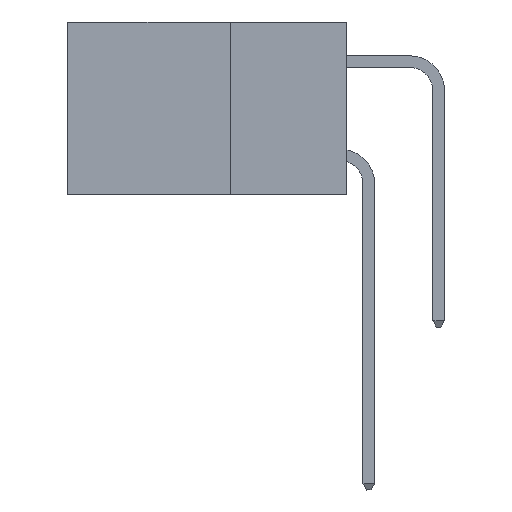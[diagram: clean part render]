
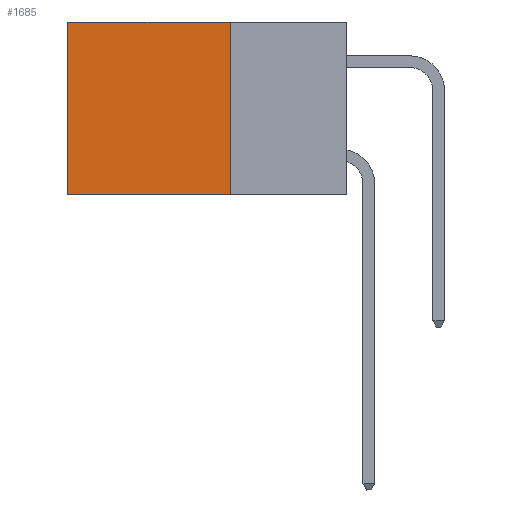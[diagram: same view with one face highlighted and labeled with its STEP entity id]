
A CAD part, left-side view. The second image highlights one B-rep face of the part: STEP entity #1685.
In plain terms, the highlighted planar face has unit normal (-1, 0, 0).
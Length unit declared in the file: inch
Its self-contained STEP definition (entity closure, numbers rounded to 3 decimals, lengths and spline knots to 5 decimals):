
#137 = VERTEX_POINT ( 'NONE', #4758 ) ;
#221 = ORIENTED_EDGE ( 'NONE', *, *, #7578, .F. ) ;
#1452 = CARTESIAN_POINT ( 'NONE',  ( 0.2875, 0.25, -0.37 ) ) ;
#1685 = ADVANCED_FACE ( 'NONE', ( #2567 ), #14187, .F. ) ;
#2338 = CARTESIAN_POINT ( 'NONE',  ( 0.2875, 0.25, 0. ) ) ;
#2486 = DIRECTION ( 'NONE',  ( 0., 0., -1. ) ) ;
#2567 = FACE_OUTER_BOUND ( 'NONE', #16604, .T. ) ;
#3935 = DIRECTION ( 'NONE',  ( 0., 1., 0. ) ) ;
#4029 = CARTESIAN_POINT ( 'NONE',  ( 0.2875, 0.25, 0. ) ) ;
#4758 = CARTESIAN_POINT ( 'NONE',  ( 0.2875, 0.6, 0. ) ) ;
#5301 = LINE ( 'NONE', #1452, #12994 ) ;
#5753 = VECTOR ( 'NONE', #16807, 39.37008 ) ;
#5781 = EDGE_CURVE ( 'NONE', #137, #7153, #13782, .T. ) ;
#5919 = CARTESIAN_POINT ( 'NONE',  ( 0.2875, 0.25, -0.37 ) ) ;
#6412 = EDGE_CURVE ( 'NONE', #6951, #137, #6416, .T. ) ;
#6416 = LINE ( 'NONE', #11622, #5753 ) ;
#6951 = VERTEX_POINT ( 'NONE', #16335 ) ;
#6966 = VECTOR ( 'NONE', #14131, 39.37008 ) ;
#7153 = VERTEX_POINT ( 'NONE', #10628 ) ;
#7578 = EDGE_CURVE ( 'NONE', #15327, #7153, #5301, .T. ) ;
#7639 = DIRECTION ( 'NONE',  ( 0., 0., -1. ) ) ;
#7728 = LINE ( 'NONE', #2338, #6966 ) ;
#8684 = AXIS2_PLACEMENT_3D ( 'NONE', #4029, #8990, #2486 ) ;
#8990 = DIRECTION ( 'NONE',  ( 1., 0., 0. ) ) ;
#10628 = CARTESIAN_POINT ( 'NONE',  ( 0.2875, 0.6, -0.37 ) ) ;
#11622 = CARTESIAN_POINT ( 'NONE',  ( 0.2875, 0.25, 0. ) ) ;
#12481 = ORIENTED_EDGE ( 'NONE', *, *, #5781, .T. ) ;
#12994 = VECTOR ( 'NONE', #3935, 39.37008 ) ;
#13051 = EDGE_CURVE ( 'NONE', #6951, #15327, #7728, .T. ) ;
#13657 = VECTOR ( 'NONE', #7639, 39.37008 ) ;
#13782 = LINE ( 'NONE', #15139, #13657 ) ;
#14131 = DIRECTION ( 'NONE',  ( 0., 0., -1. ) ) ;
#14187 = PLANE ( 'NONE',  #8684 ) ;
#15139 = CARTESIAN_POINT ( 'NONE',  ( 0.2875, 0.6, 0. ) ) ;
#15327 = VERTEX_POINT ( 'NONE', #5919 ) ;
#15936 = ORIENTED_EDGE ( 'NONE', *, *, #13051, .F. ) ;
#16335 = CARTESIAN_POINT ( 'NONE',  ( 0.2875, 0.25, 0. ) ) ;
#16604 = EDGE_LOOP ( 'NONE', ( #12481, #221, #15936, #16666 ) ) ;
#16666 = ORIENTED_EDGE ( 'NONE', *, *, #6412, .T. ) ;
#16807 = DIRECTION ( 'NONE',  ( 0., 1., 0. ) ) ;
